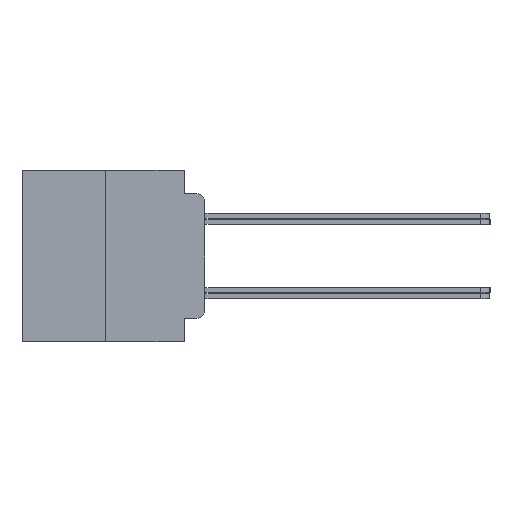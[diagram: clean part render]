
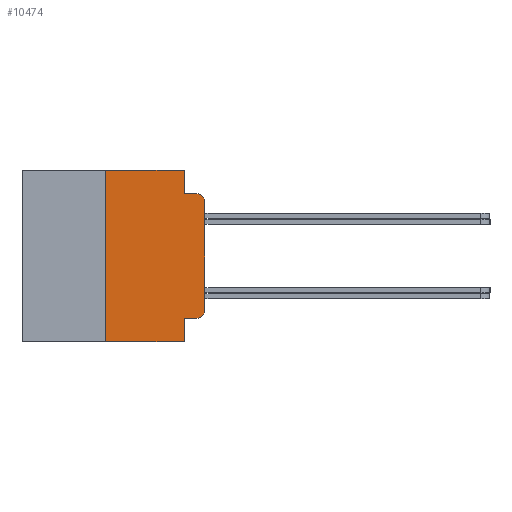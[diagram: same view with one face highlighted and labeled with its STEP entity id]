
A CAD part, left-side view. The second image highlights one B-rep face of the part: STEP entity #10474.
In plain terms, the highlighted planar face has unit normal (-1, 0, 0).
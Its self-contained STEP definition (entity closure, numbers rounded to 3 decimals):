
#826 = DIRECTION ( 'NONE',  ( 0., -1., 0. ) ) ;
#1263 = CARTESIAN_POINT ( 'NONE',  ( -75.603, 11.684, -5.486 ) ) ;
#1346 = CARTESIAN_POINT ( 'NONE',  ( -75.603, 1.295, -3.975 ) ) ;
#1634 = DIRECTION ( 'NONE',  ( 0., 0., -1. ) ) ;
#1729 = CARTESIAN_POINT ( 'NONE',  ( -75.603, 11.684, 5.486 ) ) ;
#1798 = EDGE_CURVE ( 'NONE', #9831, #16738, #3325, .T. ) ;
#1999 = AXIS2_PLACEMENT_3D ( 'NONE', #1729, #27019, #1634 ) ;
#2350 = VECTOR ( 'NONE', #4030, 1000. ) ;
#2674 = VERTEX_POINT ( 'NONE', #15322 ) ;
#2837 = VERTEX_POINT ( 'NONE', #6845 ) ;
#2907 = CARTESIAN_POINT ( 'NONE',  ( -75.603, 1.295, 3.975 ) ) ;
#2970 = ORIENTED_EDGE ( 'NONE', *, *, #6041, .T. ) ;
#3089 = VECTOR ( 'NONE', #22044, 1000. ) ;
#3138 = LINE ( 'NONE', #18133, #22516 ) ;
#3325 = LINE ( 'NONE', #28615, #24887 ) ;
#3394 = DIRECTION ( 'NONE',  ( 0., -1., 0. ) ) ;
#3537 = CARTESIAN_POINT ( 'NONE',  ( -75.603, 0., 3.467 ) ) ;
#4030 = DIRECTION ( 'NONE',  ( 0., -1., 0. ) ) ;
#4170 = CIRCLE ( 'NONE', #16345, 0.508 ) ;
#4742 = CARTESIAN_POINT ( 'NONE',  ( -75.603, 0.508, -3.467 ) ) ;
#5292 = EDGE_CURVE ( 'NONE', #18421, #9401, #21478, .T. ) ;
#6041 = EDGE_CURVE ( 'NONE', #29101, #16738, #7375, .T. ) ;
#6207 = EDGE_CURVE ( 'NONE', #25536, #9401, #4170, .T. ) ;
#6845 = CARTESIAN_POINT ( 'NONE',  ( -75.603, 6.35, 5.486 ) ) ;
#7375 = LINE ( 'NONE', #1263, #3089 ) ;
#7635 = EDGE_CURVE ( 'NONE', #19838, #25536, #3138, .T. ) ;
#8041 = VECTOR ( 'NONE', #8932, 1000. ) ;
#8433 = LINE ( 'NONE', #24735, #2350 ) ;
#8932 = DIRECTION ( 'NONE',  ( 0., 0., 1. ) ) ;
#8933 = DIRECTION ( 'NONE',  ( -1., 0., 0. ) ) ;
#9360 = ORIENTED_EDGE ( 'NONE', *, *, #21855, .F. ) ;
#9401 = VERTEX_POINT ( 'NONE', #21992 ) ;
#9452 = DIRECTION ( 'NONE',  ( -1., 0., 0. ) ) ;
#9831 = VERTEX_POINT ( 'NONE', #1346 ) ;
#10438 = VECTOR ( 'NONE', #21511, 1000. ) ;
#10474 = ADVANCED_FACE ( 'NONE', ( #17663 ), #13274, .F. ) ;
#10876 = ORIENTED_EDGE ( 'NONE', *, *, #27488, .F. ) ;
#11019 = VECTOR ( 'NONE', #3394, 1000. ) ;
#11077 = CARTESIAN_POINT ( 'NONE',  ( -75.603, 6.35, -5.486 ) ) ;
#11950 = EDGE_CURVE ( 'NONE', #13261, #19838, #14410, .T. ) ;
#13261 = VERTEX_POINT ( 'NONE', #15540 ) ;
#13274 = PLANE ( 'NONE',  #1999 ) ;
#13643 = DIRECTION ( 'NONE',  ( 0., 0., 1. ) ) ;
#14381 = CARTESIAN_POINT ( 'NONE',  ( -75.603, 11.684, 5.486 ) ) ;
#14410 = CIRCLE ( 'NONE', #18153, 0.508 ) ;
#15322 = CARTESIAN_POINT ( 'NONE',  ( -75.603, 1.295, 5.486 ) ) ;
#15378 = CARTESIAN_POINT ( 'NONE',  ( -75.603, 6.35, -5.486 ) ) ;
#15540 = CARTESIAN_POINT ( 'NONE',  ( -75.603, 0.508, -3.975 ) ) ;
#16018 = ORIENTED_EDGE ( 'NONE', *, *, #18072, .T. ) ;
#16345 = AXIS2_PLACEMENT_3D ( 'NONE', #20426, #8933, #25061 ) ;
#16738 = VERTEX_POINT ( 'NONE', #21894 ) ;
#17114 = CARTESIAN_POINT ( 'NONE',  ( -75.603, 1.295, 3.975 ) ) ;
#17242 = CARTESIAN_POINT ( 'NONE',  ( -75.603, 1.295, 0. ) ) ;
#17517 = ORIENTED_EDGE ( 'NONE', *, *, #6207, .T. ) ;
#17663 = FACE_OUTER_BOUND ( 'NONE', #18918, .T. ) ;
#18072 = EDGE_CURVE ( 'NONE', #9831, #13261, #8433, .T. ) ;
#18133 = CARTESIAN_POINT ( 'NONE',  ( -75.603, 0., 5.486 ) ) ;
#18153 = AXIS2_PLACEMENT_3D ( 'NONE', #4742, #9452, #18604 ) ;
#18421 = VERTEX_POINT ( 'NONE', #2907 ) ;
#18604 = DIRECTION ( 'NONE',  ( 0., 0., -1. ) ) ;
#18918 = EDGE_LOOP ( 'NONE', ( #16018, #19848, #27613, #17517, #28279, #23002, #10876, #9360, #2970, #20708 ) ) ;
#19838 = VERTEX_POINT ( 'NONE', #29517 ) ;
#19848 = ORIENTED_EDGE ( 'NONE', *, *, #11950, .T. ) ;
#20193 = LINE ( 'NONE', #14381, #26316 ) ;
#20426 = CARTESIAN_POINT ( 'NONE',  ( -75.603, 0.508, 3.467 ) ) ;
#20708 = ORIENTED_EDGE ( 'NONE', *, *, #1798, .F. ) ;
#21478 = LINE ( 'NONE', #17114, #11019 ) ;
#21511 = DIRECTION ( 'NONE',  ( 0., 0., -1. ) ) ;
#21855 = EDGE_CURVE ( 'NONE', #29101, #2837, #23880, .T. ) ;
#21894 = CARTESIAN_POINT ( 'NONE',  ( -75.603, 1.295, -5.486 ) ) ;
#21992 = CARTESIAN_POINT ( 'NONE',  ( -75.603, 0.508, 3.975 ) ) ;
#22044 = DIRECTION ( 'NONE',  ( 0., -1., 0. ) ) ;
#22516 = VECTOR ( 'NONE', #13643, 1000. ) ;
#23002 = ORIENTED_EDGE ( 'NONE', *, *, #24157, .F. ) ;
#23376 = LINE ( 'NONE', #17242, #10438 ) ;
#23880 = LINE ( 'NONE', #11077, #8041 ) ;
#24157 = EDGE_CURVE ( 'NONE', #2674, #18421, #23376, .T. ) ;
#24735 = CARTESIAN_POINT ( 'NONE',  ( -75.603, 1.295, -3.975 ) ) ;
#24887 = VECTOR ( 'NONE', #26219, 1000. ) ;
#25061 = DIRECTION ( 'NONE',  ( 0., 0., -1. ) ) ;
#25536 = VERTEX_POINT ( 'NONE', #3537 ) ;
#26219 = DIRECTION ( 'NONE',  ( 0., 0., -1. ) ) ;
#26316 = VECTOR ( 'NONE', #826, 1000. ) ;
#27019 = DIRECTION ( 'NONE',  ( 1., 0., 0. ) ) ;
#27488 = EDGE_CURVE ( 'NONE', #2837, #2674, #20193, .T. ) ;
#27613 = ORIENTED_EDGE ( 'NONE', *, *, #7635, .T. ) ;
#28279 = ORIENTED_EDGE ( 'NONE', *, *, #5292, .F. ) ;
#28615 = CARTESIAN_POINT ( 'NONE',  ( -75.603, 1.295, 0. ) ) ;
#29101 = VERTEX_POINT ( 'NONE', #15378 ) ;
#29517 = CARTESIAN_POINT ( 'NONE',  ( -75.603, 0., -3.467 ) ) ;
